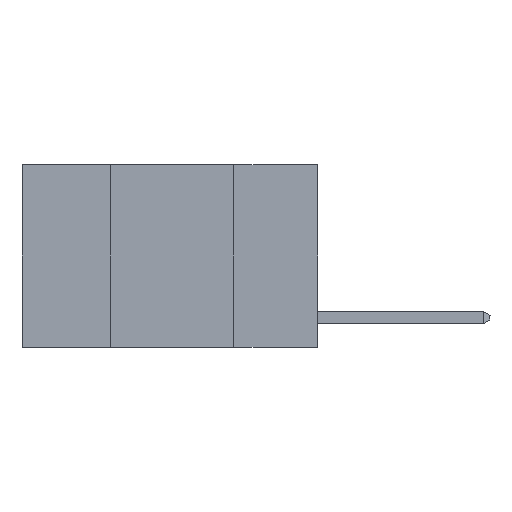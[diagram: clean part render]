
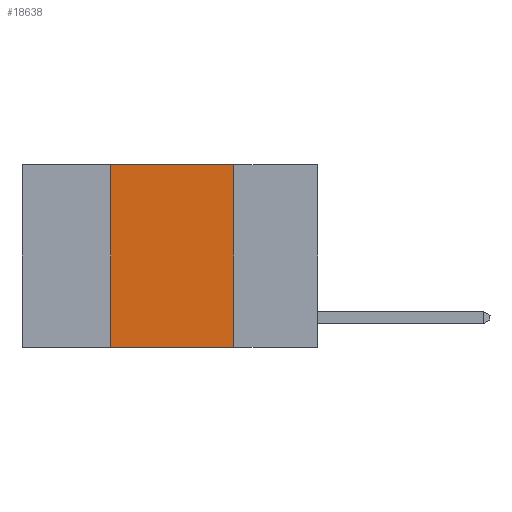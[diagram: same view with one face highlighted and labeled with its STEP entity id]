
A CAD part, left-side view. The second image highlights one B-rep face of the part: STEP entity #18638.
In plain terms, the highlighted planar face has unit normal (-1, 0, 0).
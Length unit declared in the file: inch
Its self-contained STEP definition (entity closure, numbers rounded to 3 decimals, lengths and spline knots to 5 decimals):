
#292 = ORIENTED_EDGE ( 'NONE', *, *, #14473, .F. ) ;
#727 = AXIS2_PLACEMENT_3D ( 'NONE', #2209, #14574, #8365 ) ;
#839 = DIRECTION ( 'NONE',  ( 0., -1., 0. ) ) ;
#845 = EDGE_CURVE ( 'NONE', #19389, #3754, #17767, .T. ) ;
#951 = CARTESIAN_POINT ( 'NONE',  ( 0., 0.42, 0. ) ) ;
#1108 = CARTESIAN_POINT ( 'NONE',  ( 0., 0.42, 0. ) ) ;
#2209 = CARTESIAN_POINT ( 'NONE',  ( 0., 0.6, 0. ) ) ;
#2330 = LINE ( 'NONE', #4130, #16835 ) ;
#2771 = DIRECTION ( 'NONE',  ( 0., -1., 0. ) ) ;
#3480 = CARTESIAN_POINT ( 'NONE',  ( 0., 0.17, 0. ) ) ;
#3641 = CARTESIAN_POINT ( 'NONE',  ( 0., 0.17, 0. ) ) ;
#3754 = VERTEX_POINT ( 'NONE', #951 ) ;
#4130 = CARTESIAN_POINT ( 'NONE',  ( 0., 0.6, -0.37 ) ) ;
#4480 = EDGE_CURVE ( 'NONE', #12874, #9275, #11333, .T. ) ;
#4950 = PLANE ( 'NONE',  #727 ) ;
#5862 = CARTESIAN_POINT ( 'NONE',  ( 0., 0.17, -0.37 ) ) ;
#6739 = EDGE_CURVE ( 'NONE', #19389, #9275, #2330, .T. ) ;
#7397 = VECTOR ( 'NONE', #2771, 39.37008 ) ;
#8365 = DIRECTION ( 'NONE',  ( 0., 0., -1. ) ) ;
#8709 = ORIENTED_EDGE ( 'NONE', *, *, #845, .F. ) ;
#9275 = VERTEX_POINT ( 'NONE', #5862 ) ;
#9483 = LINE ( 'NONE', #18728, #7397 ) ;
#9500 = VECTOR ( 'NONE', #17964, 39.37008 ) ;
#9678 = FACE_OUTER_BOUND ( 'NONE', #18227, .T. ) ;
#11333 = LINE ( 'NONE', #3480, #11683 ) ;
#11683 = VECTOR ( 'NONE', #19158, 39.37008 ) ;
#11713 = ORIENTED_EDGE ( 'NONE', *, *, #6739, .T. ) ;
#12874 = VERTEX_POINT ( 'NONE', #3641 ) ;
#14473 = EDGE_CURVE ( 'NONE', #3754, #12874, #9483, .T. ) ;
#14574 = DIRECTION ( 'NONE',  ( 1., 0., 0. ) ) ;
#16831 = CARTESIAN_POINT ( 'NONE',  ( 0., 0.42, -0.37 ) ) ;
#16835 = VECTOR ( 'NONE', #839, 39.37008 ) ;
#17736 = ORIENTED_EDGE ( 'NONE', *, *, #4480, .F. ) ;
#17767 = LINE ( 'NONE', #1108, #9500 ) ;
#17964 = DIRECTION ( 'NONE',  ( 0., 0., 1. ) ) ;
#18227 = EDGE_LOOP ( 'NONE', ( #17736, #292, #8709, #11713 ) ) ;
#18638 = ADVANCED_FACE ( 'NONE', ( #9678 ), #4950, .F. ) ;
#18728 = CARTESIAN_POINT ( 'NONE',  ( 0., 0.6, 0. ) ) ;
#19158 = DIRECTION ( 'NONE',  ( 0., 0., -1. ) ) ;
#19389 = VERTEX_POINT ( 'NONE', #16831 ) ;
